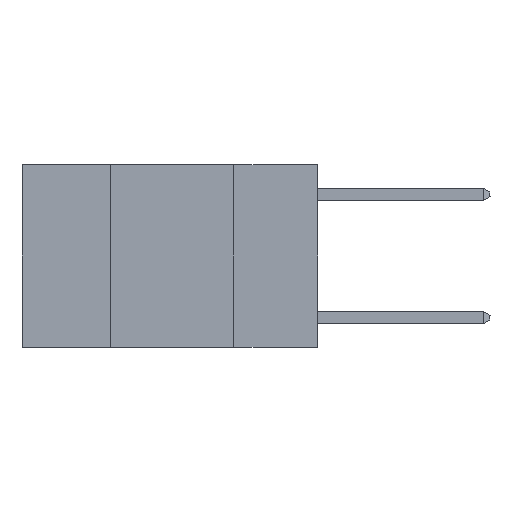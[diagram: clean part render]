
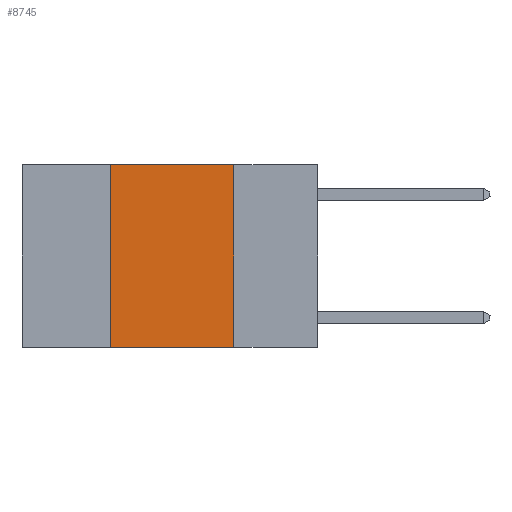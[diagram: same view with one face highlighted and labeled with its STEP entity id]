
A CAD part, left-side view. The second image highlights one B-rep face of the part: STEP entity #8745.
In plain terms, the highlighted planar face has unit normal (-1, 0, 0).
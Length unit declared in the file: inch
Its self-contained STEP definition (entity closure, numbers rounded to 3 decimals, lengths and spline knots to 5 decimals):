
#1607 = EDGE_CURVE ( 'NONE', #3610, #2530, #10323, .T. ) ;
#1656 = ORIENTED_EDGE ( 'NONE', *, *, #9020, .T. ) ;
#1691 = FACE_OUTER_BOUND ( 'NONE', #4715, .T. ) ;
#1826 = VECTOR ( 'NONE', #6029, 39.37008 ) ;
#1899 = DIRECTION ( 'NONE',  ( 0., 0., 1. ) ) ;
#2530 = VERTEX_POINT ( 'NONE', #6555 ) ;
#3602 = CARTESIAN_POINT ( 'NONE',  ( 0., 0.42, 0. ) ) ;
#3610 = VERTEX_POINT ( 'NONE', #7616 ) ;
#4035 = EDGE_CURVE ( 'NONE', #6888, #3610, #6854, .T. ) ;
#4358 = CARTESIAN_POINT ( 'NONE',  ( 0., 0.6, 0. ) ) ;
#4388 = CARTESIAN_POINT ( 'NONE',  ( 0., 0.42, -0.37 ) ) ;
#4487 = VERTEX_POINT ( 'NONE', #4388 ) ;
#4715 = EDGE_LOOP ( 'NONE', ( #8322, #9791, #5195, #1656 ) ) ;
#4756 = CARTESIAN_POINT ( 'NONE',  ( 0., 0.42, 0. ) ) ;
#4901 = DIRECTION ( 'NONE',  ( 1., 0., 0. ) ) ;
#4945 = CARTESIAN_POINT ( 'NONE',  ( 0., 0.6, 0. ) ) ;
#5080 = DIRECTION ( 'NONE',  ( 0., -1., 0. ) ) ;
#5195 = ORIENTED_EDGE ( 'NONE', *, *, #6701, .F. ) ;
#5258 = VECTOR ( 'NONE', #7978, 39.37008 ) ;
#5413 = CARTESIAN_POINT ( 'NONE',  ( 0., 0.17, 0. ) ) ;
#6029 = DIRECTION ( 'NONE',  ( 0., -1., 0. ) ) ;
#6238 = CARTESIAN_POINT ( 'NONE',  ( 0., 0.6, -0.37 ) ) ;
#6555 = CARTESIAN_POINT ( 'NONE',  ( 0., 0.17, -0.37 ) ) ;
#6701 = EDGE_CURVE ( 'NONE', #4487, #6888, #9893, .T. ) ;
#6854 = LINE ( 'NONE', #4358, #7661 ) ;
#6888 = VERTEX_POINT ( 'NONE', #4756 ) ;
#6917 = LINE ( 'NONE', #6238, #1826 ) ;
#7307 = PLANE ( 'NONE',  #8414 ) ;
#7616 = CARTESIAN_POINT ( 'NONE',  ( 0., 0.17, 0. ) ) ;
#7661 = VECTOR ( 'NONE', #5080, 39.37008 ) ;
#7978 = DIRECTION ( 'NONE',  ( 0., 0., -1. ) ) ;
#8128 = DIRECTION ( 'NONE',  ( 0., 0., -1. ) ) ;
#8322 = ORIENTED_EDGE ( 'NONE', *, *, #1607, .F. ) ;
#8414 = AXIS2_PLACEMENT_3D ( 'NONE', #4945, #4901, #8128 ) ;
#8745 = ADVANCED_FACE ( 'NONE', ( #1691 ), #7307, .F. ) ;
#9020 = EDGE_CURVE ( 'NONE', #4487, #2530, #6917, .T. ) ;
#9587 = VECTOR ( 'NONE', #1899, 39.37008 ) ;
#9791 = ORIENTED_EDGE ( 'NONE', *, *, #4035, .F. ) ;
#9893 = LINE ( 'NONE', #3602, #9587 ) ;
#10323 = LINE ( 'NONE', #5413, #5258 ) ;
